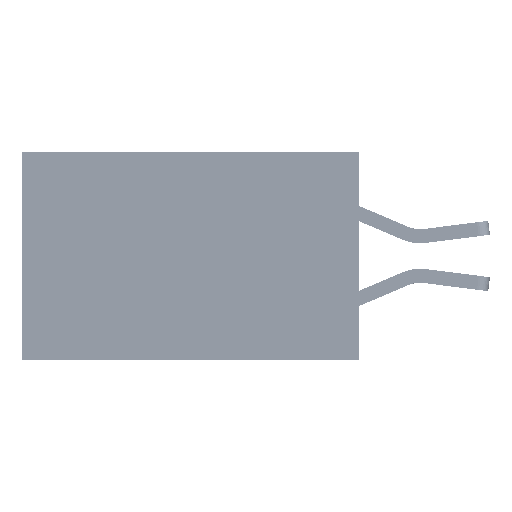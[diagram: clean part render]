
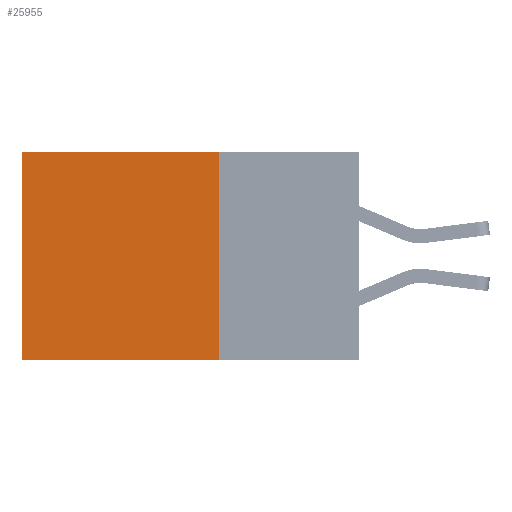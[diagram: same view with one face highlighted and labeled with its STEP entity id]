
A CAD part, left-side view. The second image highlights one B-rep face of the part: STEP entity #25955.
In plain terms, the highlighted planar face has unit normal (-1, 0, 0).
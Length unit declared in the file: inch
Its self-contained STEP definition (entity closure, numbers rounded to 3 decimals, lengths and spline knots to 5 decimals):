
#989 = DIRECTION ( 'NONE',  ( 0., 1., 0. ) ) ;
#2092 = PLANE ( 'NONE',  #5052 ) ;
#4091 = ORIENTED_EDGE ( 'NONE', *, *, #25326, .F. ) ;
#4223 = CARTESIAN_POINT ( 'NONE',  ( 0.2875, 0.25, 0. ) ) ;
#5052 = AXIS2_PLACEMENT_3D ( 'NONE', #36643, #42811, #12878 ) ;
#5139 = VECTOR ( 'NONE', #36886, 39.37008 ) ;
#5753 = ORIENTED_EDGE ( 'NONE', *, *, #41938, .T. ) ;
#6517 = EDGE_CURVE ( 'NONE', #30051, #41583, #30487, .T. ) ;
#7367 = CARTESIAN_POINT ( 'NONE',  ( 0.2875, 0.25, 0. ) ) ;
#12878 = DIRECTION ( 'NONE',  ( 0., 0., -1. ) ) ;
#14864 = VECTOR ( 'NONE', #30996, 39.37008 ) ;
#15520 = EDGE_LOOP ( 'NONE', ( #5753, #4091, #31661, #18059 ) ) ;
#18059 = ORIENTED_EDGE ( 'NONE', *, *, #22368, .T. ) ;
#18966 = CARTESIAN_POINT ( 'NONE',  ( 0.2875, 0.6, 0. ) ) ;
#20820 = CARTESIAN_POINT ( 'NONE',  ( 0.2875, 0.6, 0. ) ) ;
#21612 = VECTOR ( 'NONE', #36909, 39.37008 ) ;
#21999 = CARTESIAN_POINT ( 'NONE',  ( 0.2875, 0.6, -0.37 ) ) ;
#22368 = EDGE_CURVE ( 'NONE', #30051, #32966, #38193, .T. ) ;
#23477 = LINE ( 'NONE', #20820, #21612 ) ;
#23735 = CARTESIAN_POINT ( 'NONE',  ( 0.2875, 0.25, -0.37 ) ) ;
#24113 = CARTESIAN_POINT ( 'NONE',  ( 0.2875, 0.25, 0. ) ) ;
#24765 = VERTEX_POINT ( 'NONE', #21999 ) ;
#25326 = EDGE_CURVE ( 'NONE', #41583, #24765, #34090, .T. ) ;
#25955 = ADVANCED_FACE ( 'NONE', ( #43033 ), #2092, .F. ) ;
#28825 = VECTOR ( 'NONE', #989, 39.37008 ) ;
#30051 = VERTEX_POINT ( 'NONE', #4223 ) ;
#30487 = LINE ( 'NONE', #24113, #5139 ) ;
#30996 = DIRECTION ( 'NONE',  ( 0., 1., 0. ) ) ;
#31661 = ORIENTED_EDGE ( 'NONE', *, *, #6517, .F. ) ;
#31871 = CARTESIAN_POINT ( 'NONE',  ( 0.2875, 0.25, -0.37 ) ) ;
#32966 = VERTEX_POINT ( 'NONE', #18966 ) ;
#34090 = LINE ( 'NONE', #23735, #14864 ) ;
#36643 = CARTESIAN_POINT ( 'NONE',  ( 0.2875, 0.25, 0. ) ) ;
#36886 = DIRECTION ( 'NONE',  ( 0., 0., -1. ) ) ;
#36909 = DIRECTION ( 'NONE',  ( 0., 0., -1. ) ) ;
#38193 = LINE ( 'NONE', #7367, #28825 ) ;
#41583 = VERTEX_POINT ( 'NONE', #31871 ) ;
#41938 = EDGE_CURVE ( 'NONE', #32966, #24765, #23477, .T. ) ;
#42811 = DIRECTION ( 'NONE',  ( 1., 0., 0. ) ) ;
#43033 = FACE_OUTER_BOUND ( 'NONE', #15520, .T. ) ;
